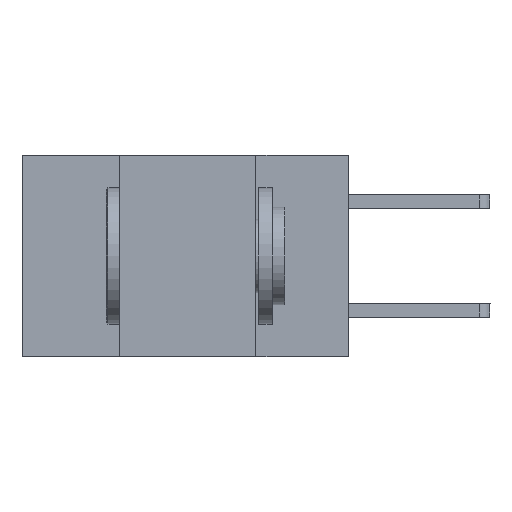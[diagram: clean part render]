
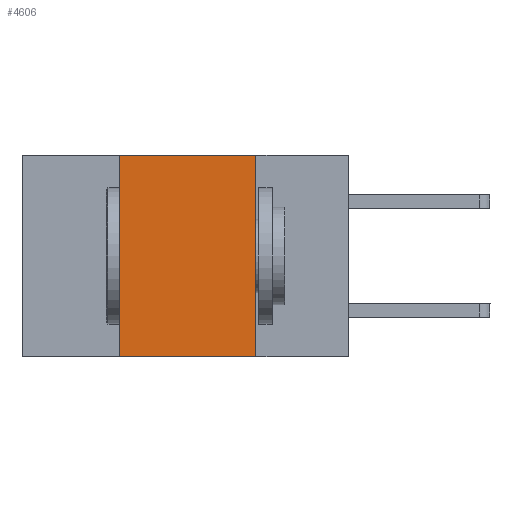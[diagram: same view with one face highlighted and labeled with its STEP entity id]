
A CAD part, left-side view. The second image highlights one B-rep face of the part: STEP entity #4606.
In plain terms, the highlighted planar face has unit normal (-1, 0, 0).
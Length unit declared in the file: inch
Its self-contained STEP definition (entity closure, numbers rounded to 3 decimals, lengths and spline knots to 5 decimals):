
#28 = EDGE_LOOP ( 'NONE', ( #5433, #8226, #1684, #3925 ) ) ;
#191 = DIRECTION ( 'NONE',  ( 0., 0., -1. ) ) ;
#590 = CARTESIAN_POINT ( 'NONE',  ( 0., 0.17, 0. ) ) ;
#709 = CARTESIAN_POINT ( 'NONE',  ( 0., 0.42, 0. ) ) ;
#787 = CARTESIAN_POINT ( 'NONE',  ( 0., 0.17, 0. ) ) ;
#821 = DIRECTION ( 'NONE',  ( 0., 0., -1. ) ) ;
#831 = CARTESIAN_POINT ( 'NONE',  ( 0., 0.42, 0. ) ) ;
#903 = VERTEX_POINT ( 'NONE', #6602 ) ;
#926 = DIRECTION ( 'NONE',  ( 0., 0., 1. ) ) ;
#1293 = VERTEX_POINT ( 'NONE', #709 ) ;
#1659 = VERTEX_POINT ( 'NONE', #3401 ) ;
#1684 = ORIENTED_EDGE ( 'NONE', *, *, #5655, .F. ) ;
#1936 = EDGE_CURVE ( 'NONE', #6766, #903, #5197, .T. ) ;
#2409 = LINE ( 'NONE', #8009, #5753 ) ;
#3401 = CARTESIAN_POINT ( 'NONE',  ( 0., 0.42, -0.37 ) ) ;
#3660 = EDGE_CURVE ( 'NONE', #1659, #903, #2409, .T. ) ;
#3691 = DIRECTION ( 'NONE',  ( 0., -1., 0. ) ) ;
#3806 = DIRECTION ( 'NONE',  ( 0., -1., 0. ) ) ;
#3925 = ORIENTED_EDGE ( 'NONE', *, *, #3660, .T. ) ;
#4334 = CARTESIAN_POINT ( 'NONE',  ( 0., 0.6, 0. ) ) ;
#4418 = LINE ( 'NONE', #6984, #6883 ) ;
#4606 = ADVANCED_FACE ( 'NONE', ( #8687 ), #8430, .F. ) ;
#5092 = AXIS2_PLACEMENT_3D ( 'NONE', #4334, #10077, #191 ) ;
#5197 = LINE ( 'NONE', #787, #7252 ) ;
#5433 = ORIENTED_EDGE ( 'NONE', *, *, #1936, .F. ) ;
#5655 = EDGE_CURVE ( 'NONE', #1659, #1293, #6070, .T. ) ;
#5753 = VECTOR ( 'NONE', #3806, 39.37008 ) ;
#5953 = VECTOR ( 'NONE', #926, 39.37008 ) ;
#6070 = LINE ( 'NONE', #831, #5953 ) ;
#6602 = CARTESIAN_POINT ( 'NONE',  ( 0., 0.17, -0.37 ) ) ;
#6766 = VERTEX_POINT ( 'NONE', #590 ) ;
#6883 = VECTOR ( 'NONE', #3691, 39.37008 ) ;
#6984 = CARTESIAN_POINT ( 'NONE',  ( 0., 0.6, 0. ) ) ;
#7252 = VECTOR ( 'NONE', #821, 39.37008 ) ;
#8009 = CARTESIAN_POINT ( 'NONE',  ( 0., 0.6, -0.37 ) ) ;
#8226 = ORIENTED_EDGE ( 'NONE', *, *, #9534, .F. ) ;
#8430 = PLANE ( 'NONE',  #5092 ) ;
#8687 = FACE_OUTER_BOUND ( 'NONE', #28, .T. ) ;
#9534 = EDGE_CURVE ( 'NONE', #1293, #6766, #4418, .T. ) ;
#10077 = DIRECTION ( 'NONE',  ( 1., 0., 0. ) ) ;
